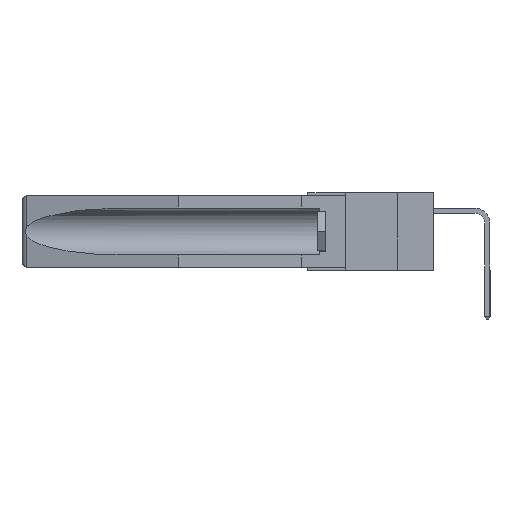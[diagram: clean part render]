
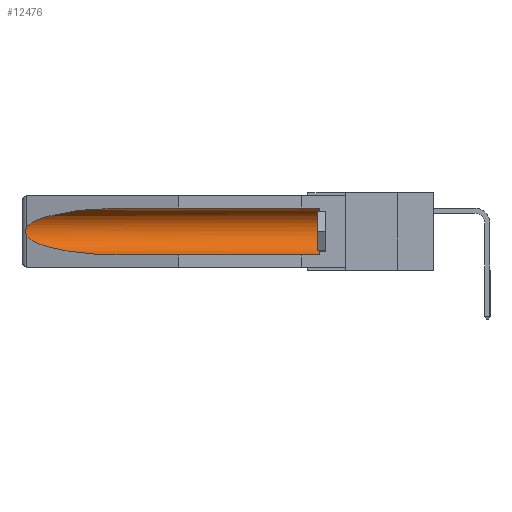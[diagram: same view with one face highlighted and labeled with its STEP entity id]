
A CAD part, left-side view. The second image highlights one B-rep face of the part: STEP entity #12476.
In plain terms, the highlighted cylindrical face has radius 2.857 mm (diameter 5.715 mm), a partial arc.
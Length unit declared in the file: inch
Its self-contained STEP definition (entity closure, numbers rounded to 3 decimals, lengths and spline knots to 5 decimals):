
#122 = CARTESIAN_POINT ( 'NONE',  ( 0.155, 0.126, -0.1715 ) ) ;
#296 = CARTESIAN_POINT ( 'NONE',  ( 0.26537, 1.52718, -0.14972 ) ) ;
#559 = CARTESIAN_POINT ( 'NONE',  ( 0.25451, 1.48313, -0.24835 ) ) ;
#837 =( BOUNDED_CURVE ( )  B_SPLINE_CURVE ( 3, ( #6601, #559, #9764, #18852 ),
 .UNSPECIFIED., .F., .F. ) 
 B_SPLINE_CURVE_WITH_KNOTS ( ( 4, 4 ),
 ( 0.1948, 1.5708 ),
 .UNSPECIFIED. ) 
 CURVE ( )  GEOMETRIC_REPRESENTATION_ITEM ( )  RATIONAL_B_SPLINE_CURVE ( ( 1., 0.848, 0.848, 1. ) ) 
 REPRESENTATION_ITEM ( '' )  );
#1095 = ORIENTED_EDGE ( 'NONE', *, *, #15714, .F. ) ;
#1812 = CARTESIAN_POINT ( 'NONE',  ( 0.155, 0.126, -0.059 ) ) ;
#1948 = EDGE_CURVE ( 'NONE', #2553, #16356, #18904, .T. ) ;
#2509 = CARTESIAN_POINT ( 'NONE',  ( 0.155, -0.30754, -0.284 ) ) ;
#2553 = VERTEX_POINT ( 'NONE', #11035 ) ;
#2920 = CARTESIAN_POINT ( 'NONE',  ( 0.25451, 1.48313, -0.09465 ) ) ;
#3531 = CARTESIAN_POINT ( 'NONE',  ( 0.155, 1.07973, -0.059 ) ) ;
#3759 = AXIS2_PLACEMENT_3D ( 'NONE', #16773, #12043, #16710 ) ;
#3856 = CARTESIAN_POINT ( 'NONE',  ( 0.155, -0.30754, -0.059 ) ) ;
#3936 = CARTESIAN_POINT ( 'NONE',  ( 0.2675, 1.53308, -0.17534 ) ) ;
#3997 = CARTESIAN_POINT ( 'NONE',  ( 0.26597, 1.5296, -0.19026 ) ) ;
#4483 = DIRECTION ( 'NONE',  ( 0., 0., 1. ) ) ;
#4905 = EDGE_CURVE ( 'NONE', #6866, #12833, #10248, .T. ) ;
#5168 = VERTEX_POINT ( 'NONE', #7560 ) ;
#5465 = CARTESIAN_POINT ( 'NONE',  ( 0.26654, 1.53092, -0.15636 ) ) ;
#5920 = LINE ( 'NONE', #2509, #10413 ) ;
#6062 = EDGE_CURVE ( 'NONE', #10025, #6866, #18198, .T. ) ;
#6216 = CARTESIAN_POINT ( 'NONE',  ( 0.26537, 1.52718, -0.14972 ) ) ;
#6601 = CARTESIAN_POINT ( 'NONE',  ( 0.26537, 1.52718, -0.19328 ) ) ;
#6866 = VERTEX_POINT ( 'NONE', #296 ) ;
#7022 = EDGE_CURVE ( 'NONE', #16356, #10025, #11383, .T. ) ;
#7560 = CARTESIAN_POINT ( 'NONE',  ( 0.155, 1.07973, -0.284 ) ) ;
#8262 = CARTESIAN_POINT ( 'NONE',  ( 0.26537, 1.52718, -0.14972 ) ) ;
#8309 = ORIENTED_EDGE ( 'NONE', *, *, #7022, .T. ) ;
#8382 = CARTESIAN_POINT ( 'NONE',  ( 0.26537, 1.52718, -0.19328 ) ) ;
#8715 = DIRECTION ( 'NONE',  ( 0., 1., 0. ) ) ;
#8739 = ORIENTED_EDGE ( 'NONE', *, *, #1948, .T. ) ;
#9085 = ORIENTED_EDGE ( 'NONE', *, *, #9953, .T. ) ;
#9115 = CARTESIAN_POINT ( 'NONE',  ( 0.155, 1.07973, -0.059 ) ) ;
#9764 = CARTESIAN_POINT ( 'NONE',  ( 0.21114, 1.30732, -0.284 ) ) ;
#9902 = CARTESIAN_POINT ( 'NONE',  ( 0.26597, 1.52961, -0.15275 ) ) ;
#9953 = EDGE_CURVE ( 'NONE', #12833, #5168, #837, .T. ) ;
#9969 = CARTESIAN_POINT ( 'NONE',  ( 0.26655, 1.53094, -0.18657 ) ) ;
#10025 = VERTEX_POINT ( 'NONE', #3531 ) ;
#10248 = B_SPLINE_CURVE_WITH_KNOTS ( 'NONE', 3,
 ( #8262, #9902, #5465, #12870, #13008, #3936, #17609, #9969, #3997, #8382 ),
 .UNSPECIFIED., .F., .F.,
 ( 4, 2, 2, 2, 4 ),
 ( 0., 0.00029, 0.00058, 0.00087, 0.00117 ),
 .UNSPECIFIED. ) ;
#10413 = VECTOR ( 'NONE', #8715, 39.37008 ) ;
#10783 = DIRECTION ( 'NONE',  ( 0., -1., 0. ) ) ;
#11035 = CARTESIAN_POINT ( 'NONE',  ( 0.155, 0.126, -0.284 ) ) ;
#11143 = AXIS2_PLACEMENT_3D ( 'NONE', #122, #10783, #4483 ) ;
#11149 = VECTOR ( 'NONE', #11423, 39.37008 ) ;
#11383 = LINE ( 'NONE', #3856, #11149 ) ;
#11423 = DIRECTION ( 'NONE',  ( 0., 1., 0. ) ) ;
#12043 = DIRECTION ( 'NONE',  ( 0., 1., 0. ) ) ;
#12476 = ADVANCED_FACE ( 'NONE', ( #18269 ), #13807, .F. ) ;
#12833 = VERTEX_POINT ( 'NONE', #14624 ) ;
#12870 = CARTESIAN_POINT ( 'NONE',  ( 0.2673, 1.5327, -0.16383 ) ) ;
#13008 = CARTESIAN_POINT ( 'NONE',  ( 0.2675, 1.53308, -0.16763 ) ) ;
#13564 = CARTESIAN_POINT ( 'NONE',  ( 0.21114, 1.30732, -0.059 ) ) ;
#13807 = CYLINDRICAL_SURFACE ( 'NONE', #3759, 0.1125 ) ;
#14544 = ORIENTED_EDGE ( 'NONE', *, *, #6062, .T. ) ;
#14624 = CARTESIAN_POINT ( 'NONE',  ( 0.26537, 1.52718, -0.19328 ) ) ;
#15498 = EDGE_LOOP ( 'NONE', ( #14544, #16934, #9085, #1095, #8739, #8309 ) ) ;
#15714 = EDGE_CURVE ( 'NONE', #2553, #5168, #5920, .T. ) ;
#16356 = VERTEX_POINT ( 'NONE', #1812 ) ;
#16710 = DIRECTION ( 'NONE',  ( 0., 0., 1. ) ) ;
#16773 = CARTESIAN_POINT ( 'NONE',  ( 0.155, -0.30754, -0.1715 ) ) ;
#16934 = ORIENTED_EDGE ( 'NONE', *, *, #4905, .T. ) ;
#17609 = CARTESIAN_POINT ( 'NONE',  ( 0.2673, 1.53269, -0.17917 ) ) ;
#18198 =( BOUNDED_CURVE ( )  B_SPLINE_CURVE ( 3, ( #9115, #13564, #2920, #6216 ),
 .UNSPECIFIED., .F., .T. ) 
 B_SPLINE_CURVE_WITH_KNOTS ( ( 4, 4 ),
 ( 4.71239, 6.08839 ),
 .UNSPECIFIED. ) 
 CURVE ( )  GEOMETRIC_REPRESENTATION_ITEM ( )  RATIONAL_B_SPLINE_CURVE ( ( 1., 0.848, 0.848, 1. ) ) 
 REPRESENTATION_ITEM ( '' )  );
#18269 = FACE_OUTER_BOUND ( 'NONE', #15498, .T. ) ;
#18852 = CARTESIAN_POINT ( 'NONE',  ( 0.155, 1.07973, -0.284 ) ) ;
#18904 = CIRCLE ( 'NONE', #11143, 0.1125 ) ;
